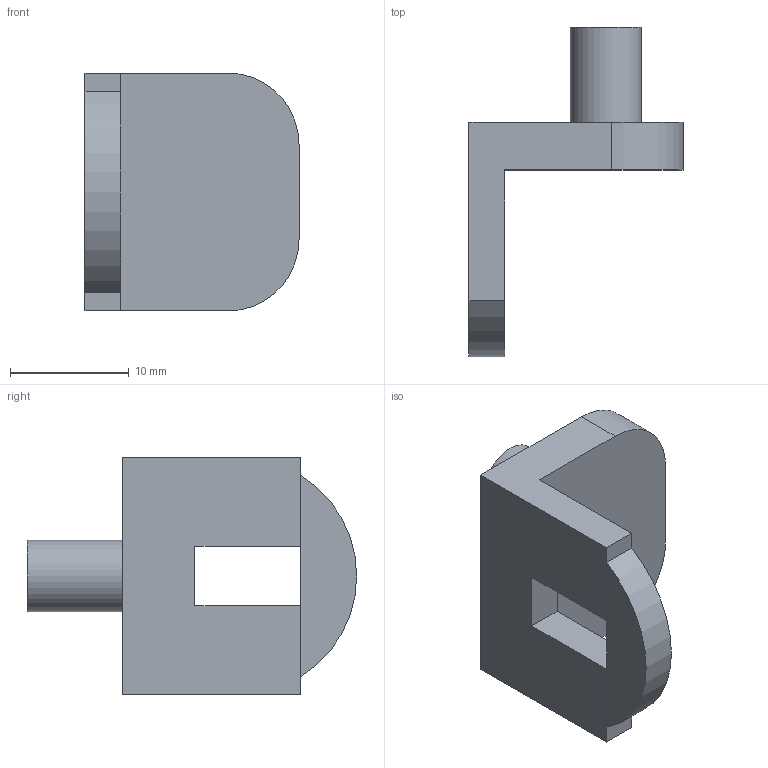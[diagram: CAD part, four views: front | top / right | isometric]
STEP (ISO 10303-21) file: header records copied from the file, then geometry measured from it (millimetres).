
FILE_DESCRIPTION(('FreeCAD Model'),'2;1');
FILE_NAME( 'AP9 ejector pivot.step', '2017-11-13T22:50:16',('Author'),(''), 'Open CASCADE STEP processor 6.8','FreeCAD','Unknown');
FILE_SCHEMA(('AUTOMOTIVE_DESIGN_CC2 { 1 2 10303 214 -1 1 5 4 }'));
Length unit declared in the file: millimetre
Products named in the file (1): Fillet001
Bounding box: 18 x 27.7 x 20 mm (x, y, z)
Volume: 2299.8 mm3; surface area: 1746.1 mm2
Topology: 1 solids, 1 shells, 20 faces, 49 edges, 30 vertices
Faces by surface type: plane 16, cylinder 4
Full cylindrical faces by diameter (mm): 6 x1
Entity records: 1232 total; most frequent: CARTESIAN_POINT 250, DIRECTION 170, LINE 109, VECTOR 109, ORIENTED_EDGE 98, PCURVE 98, DEFINITIONAL_REPRESENTATION 98, EDGE_CURVE 49
